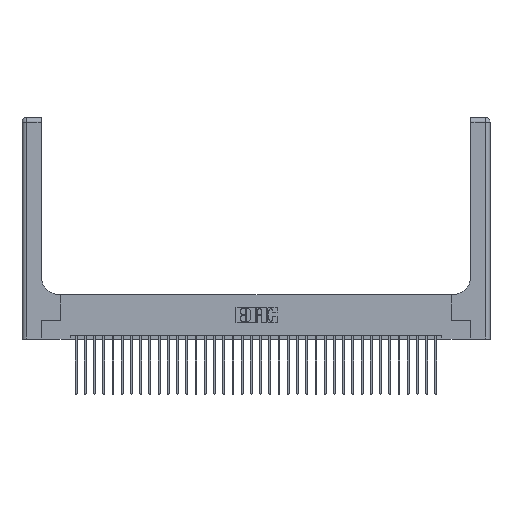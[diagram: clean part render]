
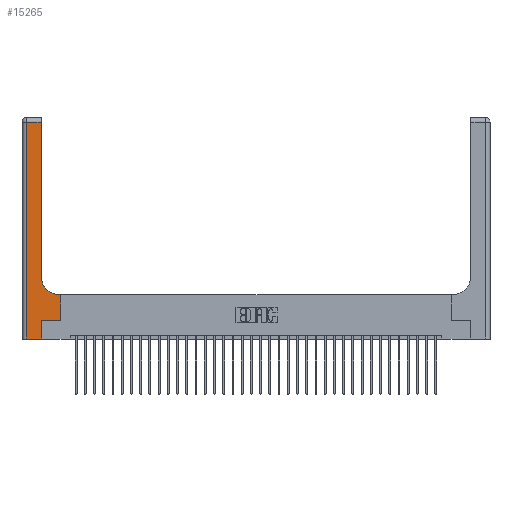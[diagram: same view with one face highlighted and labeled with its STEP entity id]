
A CAD part, top view. The second image highlights one B-rep face of the part: STEP entity #15265.
In plain terms, the highlighted planar face has unit normal (0, 0, 1).
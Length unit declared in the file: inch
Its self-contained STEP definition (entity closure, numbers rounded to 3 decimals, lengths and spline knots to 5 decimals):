
#688 = CARTESIAN_POINT ( 'NONE',  ( 0.06, 3., 0.37 ) ) ;
#1109 = ORIENTED_EDGE ( 'NONE', *, *, #22054, .T. ) ;
#1188 = ORIENTED_EDGE ( 'NONE', *, *, #7643, .T. ) ;
#1551 = LINE ( 'NONE', #9563, #30212 ) ;
#1702 = ORIENTED_EDGE ( 'NONE', *, *, #8762, .T. ) ;
#1746 = VECTOR ( 'NONE', #15772, 39.37008 ) ;
#2695 = CARTESIAN_POINT ( 'NONE',  ( 0.265, 0.25, 0.37 ) ) ;
#3470 = LINE ( 'NONE', #688, #10323 ) ;
#3582 = EDGE_CURVE ( 'NONE', #28283, #13779, #1551, .T. ) ;
#3700 = AXIS2_PLACEMENT_3D ( 'NONE', #5161, #5268, #22227 ) ;
#4155 = VECTOR ( 'NONE', #25901, 39.37008 ) ;
#4177 = ORIENTED_EDGE ( 'NONE', *, *, #20313, .T. ) ;
#4889 = VECTOR ( 'NONE', #8635, 39.37008 ) ;
#5130 = FACE_OUTER_BOUND ( 'NONE', #31278, .T. ) ;
#5161 = CARTESIAN_POINT ( 'NONE',  ( 0., 3., 0.37 ) ) ;
#5268 = DIRECTION ( 'NONE',  ( 0., 0., -1. ) ) ;
#5372 = ORIENTED_EDGE ( 'NONE', *, *, #3582, .T. ) ;
#5591 = VERTEX_POINT ( 'NONE', #11474 ) ;
#6489 = VERTEX_POINT ( 'NONE', #22175 ) ;
#7643 = EDGE_CURVE ( 'NONE', #15555, #5591, #19157, .T. ) ;
#8184 = VECTOR ( 'NONE', #8619, 39.37008 ) ;
#8387 = VERTEX_POINT ( 'NONE', #28364 ) ;
#8619 = DIRECTION ( 'NONE',  ( 0., 1., 0. ) ) ;
#8635 = DIRECTION ( 'NONE',  ( 1., 0., 0. ) ) ;
#8762 = EDGE_CURVE ( 'NONE', #30455, #9092, #3470, .T. ) ;
#9040 = LINE ( 'NONE', #2695, #27351 ) ;
#9092 = VERTEX_POINT ( 'NONE', #17078 ) ;
#9563 = CARTESIAN_POINT ( 'NONE',  ( 0.265, 0., 0.37 ) ) ;
#10323 = VECTOR ( 'NONE', #15409, 39.37008 ) ;
#10583 = DIRECTION ( 'NONE',  ( 0., 1., 0. ) ) ;
#10591 = AXIS2_PLACEMENT_3D ( 'NONE', #27307, #17600, #20042 ) ;
#10691 = EDGE_CURVE ( 'NONE', #9092, #28283, #30136, .T. ) ;
#11148 = ORIENTED_EDGE ( 'NONE', *, *, #26538, .T. ) ;
#11474 = CARTESIAN_POINT ( 'NONE',  ( 0.528, 0.6, 0.37 ) ) ;
#12193 = LINE ( 'NONE', #16493, #4155 ) ;
#13779 = VERTEX_POINT ( 'NONE', #27684 ) ;
#13826 = ORIENTED_EDGE ( 'NONE', *, *, #22396, .T. ) ;
#15265 = ADVANCED_FACE ( 'NONE', ( #5130 ), #19780, .F. ) ;
#15409 = DIRECTION ( 'NONE',  ( 0., -1., 0. ) ) ;
#15555 = VERTEX_POINT ( 'NONE', #25765 ) ;
#15772 = DIRECTION ( 'NONE',  ( -1., 0., 0. ) ) ;
#16493 = CARTESIAN_POINT ( 'NONE',  ( 0., 2.94, 0.37 ) ) ;
#16943 = LINE ( 'NONE', #25567, #8184 ) ;
#17078 = CARTESIAN_POINT ( 'NONE',  ( 0.06, 0., 0.37 ) ) ;
#17600 = DIRECTION ( 'NONE',  ( 0., 0., -1. ) ) ;
#18024 = CARTESIAN_POINT ( 'NONE',  ( 0.26, 0.6, 0.37 ) ) ;
#19157 = LINE ( 'NONE', #28184, #30286 ) ;
#19780 = PLANE ( 'NONE',  #3700 ) ;
#20042 = DIRECTION ( 'NONE',  ( 1., 0., 0. ) ) ;
#20313 = EDGE_CURVE ( 'NONE', #6489, #30455, #12193, .T. ) ;
#22054 = EDGE_CURVE ( 'NONE', #5591, #8387, #24306, .T. ) ;
#22175 = CARTESIAN_POINT ( 'NONE',  ( 0.26, 2.94, 0.37 ) ) ;
#22227 = DIRECTION ( 'NONE',  ( -1., 0., 0. ) ) ;
#22396 = EDGE_CURVE ( 'NONE', #13779, #15555, #9040, .T. ) ;
#23098 = EDGE_CURVE ( 'NONE', #8387, #24703, #25800, .T. ) ;
#24306 = LINE ( 'NONE', #18024, #1746 ) ;
#24671 = DIRECTION ( 'NONE',  ( 1., 0., 0. ) ) ;
#24703 = VERTEX_POINT ( 'NONE', #28635 ) ;
#25567 = CARTESIAN_POINT ( 'NONE',  ( 0.26, 3., 0.37 ) ) ;
#25765 = CARTESIAN_POINT ( 'NONE',  ( 0.528, 0.25, 0.37 ) ) ;
#25800 = CIRCLE ( 'NONE', #10591, 0.25 ) ;
#25805 = CARTESIAN_POINT ( 'NONE',  ( 0., 0., 0.37 ) ) ;
#25901 = DIRECTION ( 'NONE',  ( -1., 0., 0. ) ) ;
#26538 = EDGE_CURVE ( 'NONE', #24703, #6489, #16943, .T. ) ;
#26662 = DIRECTION ( 'NONE',  ( 0., 1., 0. ) ) ;
#27307 = CARTESIAN_POINT ( 'NONE',  ( 0.51, 0.85, 0.37 ) ) ;
#27351 = VECTOR ( 'NONE', #24671, 39.37008 ) ;
#27550 = CARTESIAN_POINT ( 'NONE',  ( 0.06, 2.94, 0.37 ) ) ;
#27684 = CARTESIAN_POINT ( 'NONE',  ( 0.265, 0.25, 0.37 ) ) ;
#28184 = CARTESIAN_POINT ( 'NONE',  ( 0.528, 0.25, 0.37 ) ) ;
#28283 = VERTEX_POINT ( 'NONE', #31081 ) ;
#28364 = CARTESIAN_POINT ( 'NONE',  ( 0.51, 0.6, 0.37 ) ) ;
#28635 = CARTESIAN_POINT ( 'NONE',  ( 0.26, 0.85, 0.37 ) ) ;
#29959 = ORIENTED_EDGE ( 'NONE', *, *, #23098, .T. ) ;
#30136 = LINE ( 'NONE', #25805, #4889 ) ;
#30212 = VECTOR ( 'NONE', #10583, 39.37008 ) ;
#30286 = VECTOR ( 'NONE', #26662, 39.37008 ) ;
#30455 = VERTEX_POINT ( 'NONE', #27550 ) ;
#30667 = ORIENTED_EDGE ( 'NONE', *, *, #10691, .T. ) ;
#31081 = CARTESIAN_POINT ( 'NONE',  ( 0.265, 0., 0.37 ) ) ;
#31278 = EDGE_LOOP ( 'NONE', ( #11148, #4177, #1702, #30667, #5372, #13826, #1188, #1109, #29959 ) ) ;
